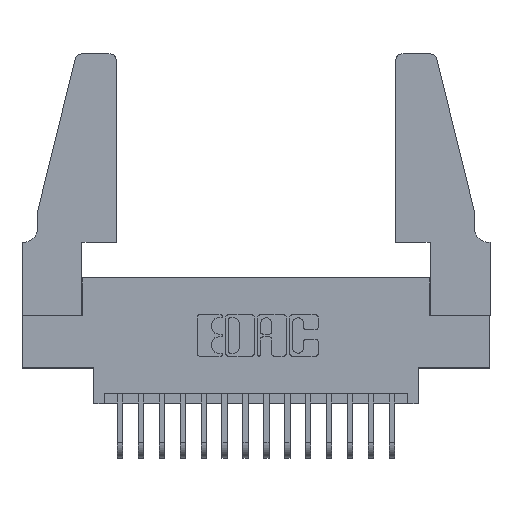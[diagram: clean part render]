
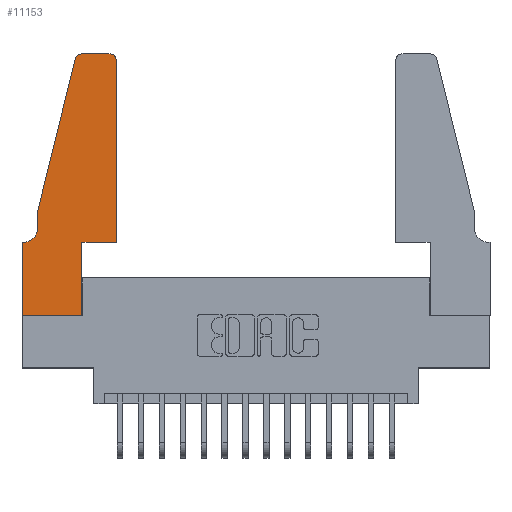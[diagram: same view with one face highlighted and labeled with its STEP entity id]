
A CAD part, top view. The second image highlights one B-rep face of the part: STEP entity #11153.
In plain terms, the highlighted planar face has unit normal (0, 0, 1).
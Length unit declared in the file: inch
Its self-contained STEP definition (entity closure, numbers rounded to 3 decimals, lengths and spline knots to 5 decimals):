
#99 = VECTOR ( 'NONE', #7610, 39.37008 ) ;
#468 = ORIENTED_EDGE ( 'NONE', *, *, #6309, .T. ) ;
#554 = DIRECTION ( 'NONE',  ( -0.239, -0.971, 0. ) ) ;
#762 = EDGE_CURVE ( 'NONE', #3032, #15030, #5629, .T. ) ;
#1415 = CARTESIAN_POINT ( 'NONE',  ( 0.0755, 0.42, 0.37 ) ) ;
#1593 = EDGE_CURVE ( 'NONE', #15030, #13365, #6436, .T. ) ;
#1623 = DIRECTION ( 'NONE',  ( 0., 0., -1. ) ) ;
#1643 = CARTESIAN_POINT ( 'NONE',  ( 0.284, 1.25, 0.37 ) ) ;
#1644 = VECTOR ( 'NONE', #15494, 39.37008 ) ;
#2052 = VECTOR ( 'NONE', #16287, 39.37008 ) ;
#2076 = EDGE_CURVE ( 'NONE', #13241, #10299, #6820, .T. ) ;
#2365 = CARTESIAN_POINT ( 'NONE',  ( 0.2865, 0.35, 0.37 ) ) ;
#2666 = ORIENTED_EDGE ( 'NONE', *, *, #9092, .T. ) ;
#2773 = EDGE_CURVE ( 'NONE', #12424, #16068, #9192, .T. ) ;
#2875 = VECTOR ( 'NONE', #15444, 39.37008 ) ;
#3032 = VERTEX_POINT ( 'NONE', #5399 ) ;
#3325 = CARTESIAN_POINT ( 'NONE',  ( 0., 0.35, 0.37 ) ) ;
#3815 = DIRECTION ( 'NONE',  ( 1., 0., 0. ) ) ;
#4379 = EDGE_LOOP ( 'NONE', ( #11022, #5644, #2666, #11489, #12043, #468, #12930, #8118, #9909, #12180, #12940, #12733 ) ) ;
#4414 = VECTOR ( 'NONE', #10283, 39.37008 ) ;
#4603 = AXIS2_PLACEMENT_3D ( 'NONE', #5849, #15001, #16341 ) ;
#5173 = LINE ( 'NONE', #7922, #1644 ) ;
#5179 = VERTEX_POINT ( 'NONE', #3325 ) ;
#5320 = CARTESIAN_POINT ( 'NONE',  ( 0.4205, 1.25, 0.37 ) ) ;
#5399 = CARTESIAN_POINT ( 'NONE',  ( 0.4505, 1.22, 0.37 ) ) ;
#5484 = EDGE_CURVE ( 'NONE', #9166, #12424, #7116, .T. ) ;
#5591 = VECTOR ( 'NONE', #11487, 39.37008 ) ;
#5629 = CIRCLE ( 'NONE', #4603, 0.03 ) ;
#5644 = ORIENTED_EDGE ( 'NONE', *, *, #10325, .T. ) ;
#5809 = DIRECTION ( 'NONE',  ( -1., 0., 0. ) ) ;
#5849 = CARTESIAN_POINT ( 'NONE',  ( 0.4205, 1.22, 0.37 ) ) ;
#5969 = AXIS2_PLACEMENT_3D ( 'NONE', #16040, #1623, #5809 ) ;
#6074 = CARTESIAN_POINT ( 'NONE',  ( 0.0055, 0.35, 0.37 ) ) ;
#6195 = DIRECTION ( 'NONE',  ( 0., 0., 1. ) ) ;
#6309 = EDGE_CURVE ( 'NONE', #10299, #5179, #5173, .T. ) ;
#6341 = CARTESIAN_POINT ( 'NONE',  ( 0.4505, 0.35, 0.37 ) ) ;
#6345 = LINE ( 'NONE', #16036, #14071 ) ;
#6436 = LINE ( 'NONE', #11507, #2875 ) ;
#6820 = CIRCLE ( 'NONE', #5969, 0.07 ) ;
#7116 = LINE ( 'NONE', #12659, #99 ) ;
#7183 = AXIS2_PLACEMENT_3D ( 'NONE', #7742, #11579, #3815 ) ;
#7610 = DIRECTION ( 'NONE',  ( 0., 1., 0. ) ) ;
#7742 = CARTESIAN_POINT ( 'NONE',  ( 0., 0.35, 0.37 ) ) ;
#7760 = LINE ( 'NONE', #11692, #14115 ) ;
#7803 = CARTESIAN_POINT ( 'NONE',  ( 0.25487, 1.22718, 0.37 ) ) ;
#7922 = CARTESIAN_POINT ( 'NONE',  ( 0.0755, 0.35, 0.37 ) ) ;
#8107 = CARTESIAN_POINT ( 'NONE',  ( 0., 0., 0.37 ) ) ;
#8118 = ORIENTED_EDGE ( 'NONE', *, *, #10083, .T. ) ;
#8395 = CARTESIAN_POINT ( 'NONE',  ( 0., 0., 0.37 ) ) ;
#8684 = CIRCLE ( 'NONE', #13018, 0.03 ) ;
#9024 = PLANE ( 'NONE',  #7183 ) ;
#9092 = EDGE_CURVE ( 'NONE', #11352, #11768, #6345, .T. ) ;
#9166 = VERTEX_POINT ( 'NONE', #16136 ) ;
#9192 = LINE ( 'NONE', #12501, #2052 ) ;
#9468 = FACE_OUTER_BOUND ( 'NONE', #4379, .T. ) ;
#9906 = EDGE_CURVE ( 'NONE', #5179, #10842, #11289, .T. ) ;
#9909 = ORIENTED_EDGE ( 'NONE', *, *, #5484, .T. ) ;
#10083 = EDGE_CURVE ( 'NONE', #10842, #9166, #11884, .T. ) ;
#10265 = CARTESIAN_POINT ( 'NONE',  ( 0.0755, 0.5, 0.37 ) ) ;
#10283 = DIRECTION ( 'NONE',  ( 0., -1., 0. ) ) ;
#10299 = VERTEX_POINT ( 'NONE', #6074 ) ;
#10325 = EDGE_CURVE ( 'NONE', #13365, #11352, #8684, .T. ) ;
#10670 = DIRECTION ( 'NONE',  ( 1., 0., 0. ) ) ;
#10842 = VERTEX_POINT ( 'NONE', #8395 ) ;
#11022 = ORIENTED_EDGE ( 'NONE', *, *, #1593, .T. ) ;
#11153 = ADVANCED_FACE ( 'NONE', ( #9468 ), #9024, .T. ) ;
#11289 = LINE ( 'NONE', #16513, #4414 ) ;
#11352 = VERTEX_POINT ( 'NONE', #7803 ) ;
#11401 = CARTESIAN_POINT ( 'NONE',  ( 0.0755, 0.5, 0.37 ) ) ;
#11487 = DIRECTION ( 'NONE',  ( 0., -1., 0. ) ) ;
#11489 = ORIENTED_EDGE ( 'NONE', *, *, #12478, .T. ) ;
#11507 = CARTESIAN_POINT ( 'NONE',  ( 0.2605, 1.25, 0.37 ) ) ;
#11579 = DIRECTION ( 'NONE',  ( 0., 0., 1. ) ) ;
#11692 = CARTESIAN_POINT ( 'NONE',  ( 0.4505, 0.35, 0.37 ) ) ;
#11768 = VERTEX_POINT ( 'NONE', #11401 ) ;
#11884 = LINE ( 'NONE', #8107, #12277 ) ;
#12000 = LINE ( 'NONE', #10265, #5591 ) ;
#12043 = ORIENTED_EDGE ( 'NONE', *, *, #2076, .T. ) ;
#12180 = ORIENTED_EDGE ( 'NONE', *, *, #2773, .T. ) ;
#12277 = VECTOR ( 'NONE', #10670, 39.37008 ) ;
#12424 = VERTEX_POINT ( 'NONE', #2365 ) ;
#12478 = EDGE_CURVE ( 'NONE', #11768, #13241, #12000, .T. ) ;
#12501 = CARTESIAN_POINT ( 'NONE',  ( 0.4505, 0.35, 0.37 ) ) ;
#12659 = CARTESIAN_POINT ( 'NONE',  ( 0.2865, 0.35, 0.37 ) ) ;
#12733 = ORIENTED_EDGE ( 'NONE', *, *, #762, .T. ) ;
#12930 = ORIENTED_EDGE ( 'NONE', *, *, #9906, .T. ) ;
#12940 = ORIENTED_EDGE ( 'NONE', *, *, #13196, .T. ) ;
#12954 = DIRECTION ( 'NONE',  ( 0., 1., 0. ) ) ;
#13018 = AXIS2_PLACEMENT_3D ( 'NONE', #13811, #6195, #15057 ) ;
#13196 = EDGE_CURVE ( 'NONE', #16068, #3032, #7760, .T. ) ;
#13241 = VERTEX_POINT ( 'NONE', #1415 ) ;
#13365 = VERTEX_POINT ( 'NONE', #1643 ) ;
#13811 = CARTESIAN_POINT ( 'NONE',  ( 0.284, 1.22, 0.37 ) ) ;
#14071 = VECTOR ( 'NONE', #554, 39.37008 ) ;
#14115 = VECTOR ( 'NONE', #12954, 39.37008 ) ;
#15001 = DIRECTION ( 'NONE',  ( 0., 0., 1. ) ) ;
#15030 = VERTEX_POINT ( 'NONE', #5320 ) ;
#15057 = DIRECTION ( 'NONE',  ( 1., 0., 0. ) ) ;
#15444 = DIRECTION ( 'NONE',  ( -1., 0., 0. ) ) ;
#15494 = DIRECTION ( 'NONE',  ( -1., 0., 0. ) ) ;
#16036 = CARTESIAN_POINT ( 'NONE',  ( 0.0755, 0.5, 0.37 ) ) ;
#16040 = CARTESIAN_POINT ( 'NONE',  ( 0.0055, 0.42, 0.37 ) ) ;
#16068 = VERTEX_POINT ( 'NONE', #6341 ) ;
#16136 = CARTESIAN_POINT ( 'NONE',  ( 0.2865, 0., 0.37 ) ) ;
#16287 = DIRECTION ( 'NONE',  ( 1., 0., 0. ) ) ;
#16341 = DIRECTION ( 'NONE',  ( 1., 0., 0. ) ) ;
#16513 = CARTESIAN_POINT ( 'NONE',  ( 0., 0., 0.37 ) ) ;
